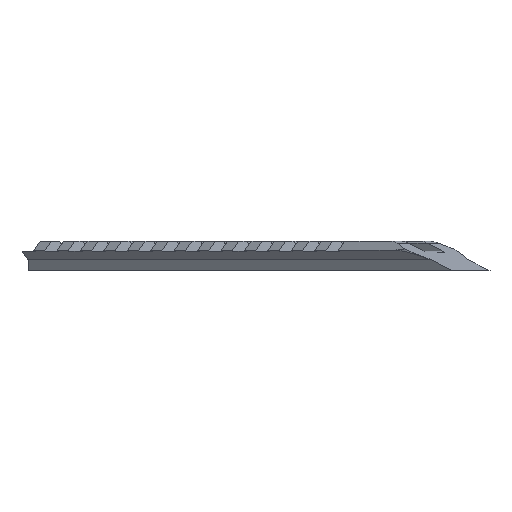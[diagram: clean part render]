
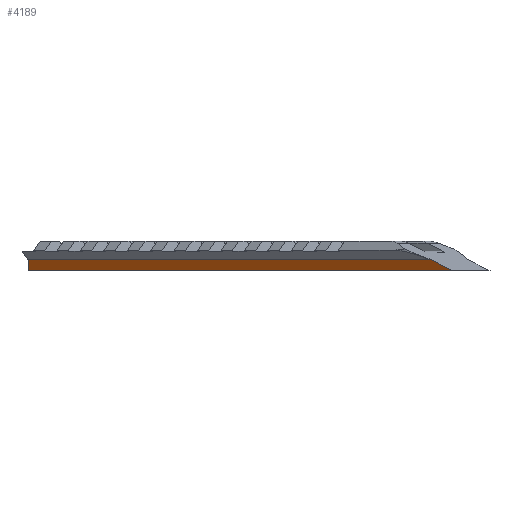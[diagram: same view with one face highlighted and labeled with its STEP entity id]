
A CAD part, front view. The second image highlights one B-rep face of the part: STEP entity #4189.
In plain terms, the highlighted planar face has unit normal (-0.707, -0.707, 0).
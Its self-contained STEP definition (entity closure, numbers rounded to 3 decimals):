
#236=PLANE('',#4462);
#445=FACE_OUTER_BOUND('',#680,.T.);
#680=EDGE_LOOP('',(#3954,#3955,#3956,#3957));
#688=LINE('',#5546,#1227);
#714=LINE('',#5675,#1253);
#717=LINE('',#5698,#1256);
#778=LINE('',#5828,#1317);
#1227=VECTOR('',#4482,10.);
#1253=VECTOR('',#4626,10.);
#1256=VECTOR('',#4649,10.);
#1317=VECTOR('',#4728,10.);
#1808=VERTEX_POINT('',#5543);
#1809=VERTEX_POINT('',#5545);
#1853=VERTEX_POINT('',#5672);
#1863=VERTEX_POINT('',#5697);
#2201=EDGE_CURVE('',#1809,#1808,#688,.T.);
#2261=EDGE_CURVE('',#1853,#1809,#714,.T.);
#2272=EDGE_CURVE('',#1863,#1853,#717,.T.);
#2338=EDGE_CURVE('',#1863,#1808,#778,.T.);
#3954=ORIENTED_EDGE('',*,*,#2261,.T.);
#3955=ORIENTED_EDGE('',*,*,#2201,.T.);
#3956=ORIENTED_EDGE('',*,*,#2338,.F.);
#3957=ORIENTED_EDGE('',*,*,#2272,.T.);
#4189=ADVANCED_FACE('',(#445),#236,.T.);
#4462=AXIS2_PLACEMENT_3D('',#6712,#5520,#5521);
#4482=DIRECTION('',(-0.664,0.664,0.345));
#4626=DIRECTION('',(0.707,-0.707,0.));
#4649=DIRECTION('',(0.,0.,-1.));
#4728=DIRECTION('',(0.707,-0.707,0.));
#5520=DIRECTION('center_axis',(-0.707,-0.707,0.));
#5521=DIRECTION('ref_axis',(0.,0.,-1.));
#5543=CARTESIAN_POINT('',(244.203,5.119,154.672));
#5545=CARTESIAN_POINT('',(250.953,-1.632,151.162));
#5546=CARTESIAN_POINT('',(120.419,128.902,219.047));
#5672=CARTESIAN_POINT('',(122.883,126.439,151.162));
#5675=CARTESIAN_POINT('',(53.687,195.635,151.162));
#5697=CARTESIAN_POINT('',(122.883,126.439,154.672));
#5698=CARTESIAN_POINT('',(122.883,126.439,154.045));
#5828=CARTESIAN_POINT('',(115.812,133.51,154.672));
#6712=CARTESIAN_POINT('Origin',(-18.538,267.86,154.672));
